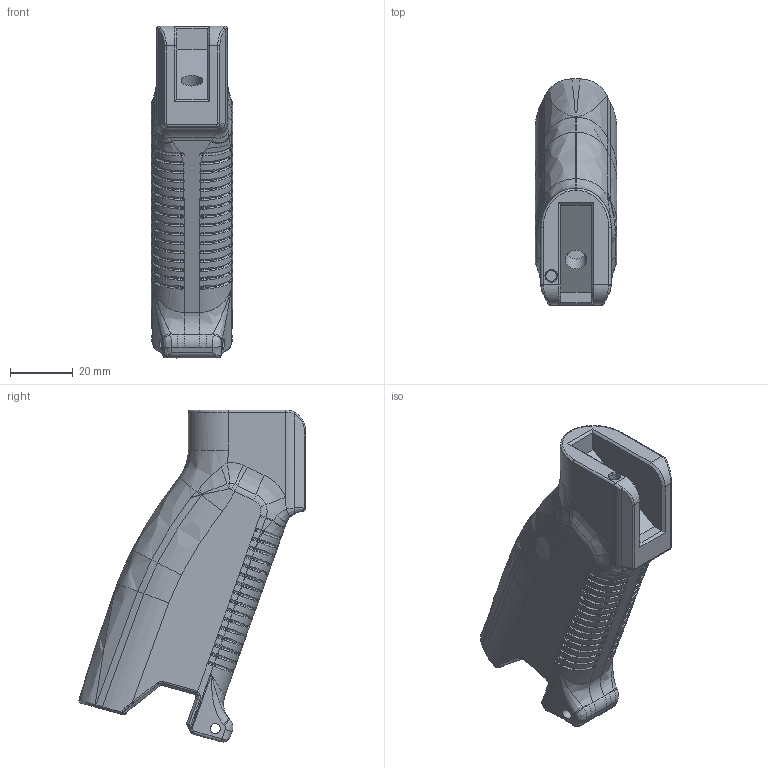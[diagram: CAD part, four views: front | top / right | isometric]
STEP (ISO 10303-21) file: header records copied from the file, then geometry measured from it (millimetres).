
FILE_DESCRIPTION(/* description */ (''),/* implementation_level */ '2;1');
FILE_NAME(/* name */ 'Textured Grip Body.step',/* time_stamp */ '2021-05-07T03:05:50-04:00',/* author */ (''),/* organization */ (''),/* preprocessor_version */ 'ST-DEVELOPER v18.1',/* originating_system */ 'Autodesk Translation Framework v10.6.0.1341',/* authorisation */ '');
FILE_SCHEMA (('AUTOMOTIVE_DESIGN { 1 0 10303 214 3 1 1 }'));
Products named in the file (1): Textured Grip Body
Bounding box: 25.93 x 72.09 x 105.63 mm (x, y, z)
Volume: 41067.1 mm3; surface area: 22437.3 mm2
Topology: 1 solids, 1 shells, 1060 faces, 2731 edges, 1654 vertices
Faces by surface type: bspline 384, cylinder 319, plane 202, torus 141, cone 12, sphere 2
Full cylindrical faces by diameter (mm): 3.2 x2, 3.4 x1, 6.8 x1
Entity records: 46384 total; most frequent: CARTESIAN_POINT 23632, ORIENTED_EDGE 5422, DIRECTION 3774, EDGE_CURVE 2711, VERTEX_POINT 1654, AXIS2_PLACEMENT_3D 1567, B_SPLINE_CURVE_WITH_KNOTS 1178, EDGE_LOOP 1067
